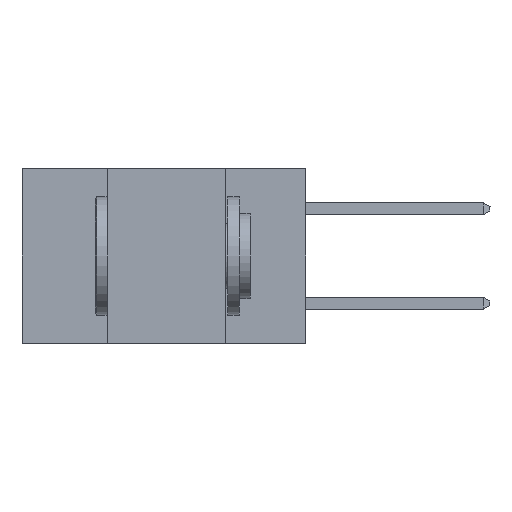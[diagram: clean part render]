
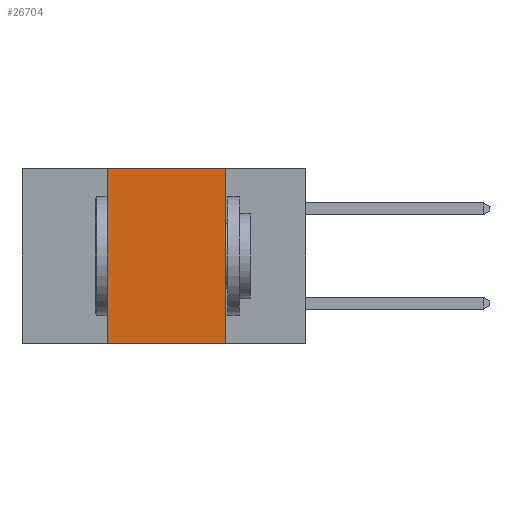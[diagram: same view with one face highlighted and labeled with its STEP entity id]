
A CAD part, left-side view. The second image highlights one B-rep face of the part: STEP entity #26704.
In plain terms, the highlighted planar face has unit normal (-1, 0, 0).
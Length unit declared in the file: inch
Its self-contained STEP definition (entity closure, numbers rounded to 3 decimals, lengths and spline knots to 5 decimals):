
#282 = DIRECTION ( 'NONE',  ( 0., -1., 0. ) ) ;
#643 = EDGE_CURVE ( 'NONE', #12140, #18357, #7273, .T. ) ;
#1161 = FACE_OUTER_BOUND ( 'NONE', #23128, .T. ) ;
#1569 = ORIENTED_EDGE ( 'NONE', *, *, #25692, .F. ) ;
#1596 = VECTOR ( 'NONE', #25094, 39.37008 ) ;
#2373 = CARTESIAN_POINT ( 'NONE',  ( 0., 0.17, 0. ) ) ;
#3429 = VERTEX_POINT ( 'NONE', #2373 ) ;
#3551 = VECTOR ( 'NONE', #26641, 39.37008 ) ;
#3793 = PLANE ( 'NONE',  #25845 ) ;
#3874 = DIRECTION ( 'NONE',  ( 1., 0., 0. ) ) ;
#6108 = VERTEX_POINT ( 'NONE', #26125 ) ;
#7273 = LINE ( 'NONE', #9166, #17965 ) ;
#8370 = EDGE_CURVE ( 'NONE', #6108, #3429, #15116, .T. ) ;
#9166 = CARTESIAN_POINT ( 'NONE',  ( 0., 0.6, -0.37 ) ) ;
#12140 = VERTEX_POINT ( 'NONE', #17579 ) ;
#14001 = CARTESIAN_POINT ( 'NONE',  ( 0., 0.6, 0. ) ) ;
#14469 = CARTESIAN_POINT ( 'NONE',  ( 0., 0.6, 0. ) ) ;
#14676 = ORIENTED_EDGE ( 'NONE', *, *, #8370, .F. ) ;
#15116 = LINE ( 'NONE', #14001, #20216 ) ;
#16439 = EDGE_CURVE ( 'NONE', #3429, #18357, #18704, .T. ) ;
#16610 = ORIENTED_EDGE ( 'NONE', *, *, #643, .T. ) ;
#17579 = CARTESIAN_POINT ( 'NONE',  ( 0., 0.42, -0.37 ) ) ;
#17965 = VECTOR ( 'NONE', #282, 39.37008 ) ;
#18357 = VERTEX_POINT ( 'NONE', #24817 ) ;
#18704 = LINE ( 'NONE', #22934, #1596 ) ;
#18828 = DIRECTION ( 'NONE',  ( 0., 0., -1. ) ) ;
#19864 = ORIENTED_EDGE ( 'NONE', *, *, #16439, .F. ) ;
#20133 = CARTESIAN_POINT ( 'NONE',  ( 0., 0.42, -0.37 ) ) ;
#20216 = VECTOR ( 'NONE', #24897, 39.37008 ) ;
#22934 = CARTESIAN_POINT ( 'NONE',  ( 0., 0.17, -0.37 ) ) ;
#23128 = EDGE_LOOP ( 'NONE', ( #19864, #14676, #1569, #16610 ) ) ;
#24817 = CARTESIAN_POINT ( 'NONE',  ( 0., 0.17, -0.37 ) ) ;
#24897 = DIRECTION ( 'NONE',  ( 0., -1., 0. ) ) ;
#25094 = DIRECTION ( 'NONE',  ( 0., 0., -1. ) ) ;
#25692 = EDGE_CURVE ( 'NONE', #12140, #6108, #26395, .T. ) ;
#25845 = AXIS2_PLACEMENT_3D ( 'NONE', #14469, #3874, #18828 ) ;
#26125 = CARTESIAN_POINT ( 'NONE',  ( 0., 0.42, 0. ) ) ;
#26395 = LINE ( 'NONE', #20133, #3551 ) ;
#26641 = DIRECTION ( 'NONE',  ( 0., 0., 1. ) ) ;
#26704 = ADVANCED_FACE ( 'NONE', ( #1161 ), #3793, .F. ) ;
